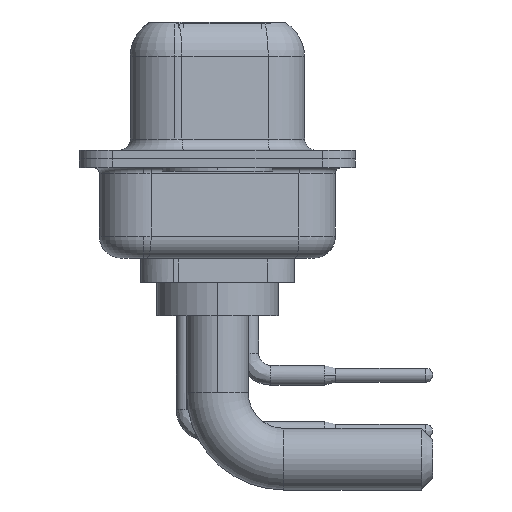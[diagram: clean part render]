
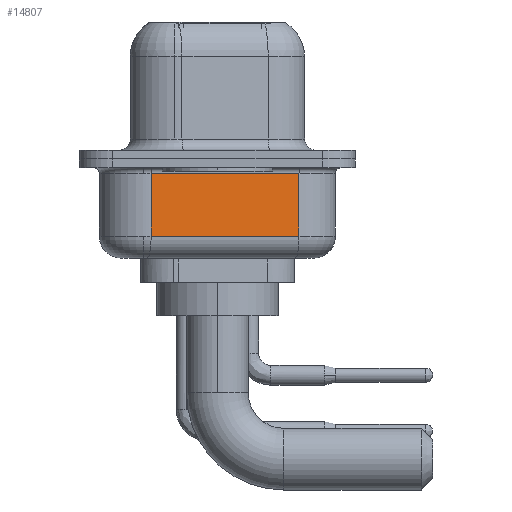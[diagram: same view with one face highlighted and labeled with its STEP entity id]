
A CAD part, left-side view. The second image highlights one B-rep face of the part: STEP entity #14807.
In plain terms, the highlighted planar face has unit normal (-0.985, -0.174, 0).
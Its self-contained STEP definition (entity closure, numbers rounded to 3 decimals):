
#488 = EDGE_CURVE ( 'NONE', #4602, #17712, #18403, .T. ) ;
#662 = LINE ( 'NONE', #10175, #16538 ) ;
#793 = AXIS2_PLACEMENT_3D ( 'NONE', #4955, #11199, #7824 ) ;
#2160 = CARTESIAN_POINT ( 'NONE',  ( 2.88, 3.003, -3.5 ) ) ;
#2682 = EDGE_CURVE ( 'NONE', #2698, #17712, #13853, .T. ) ;
#2698 = VERTEX_POINT ( 'NONE', #7511 ) ;
#3699 = LINE ( 'NONE', #5219, #5536 ) ;
#4392 = CARTESIAN_POINT ( 'NONE',  ( 2.88, 3.003, -4.5 ) ) ;
#4602 = VERTEX_POINT ( 'NONE', #2160 ) ;
#4955 = CARTESIAN_POINT ( 'NONE',  ( 2.88, 3.003, -4.5 ) ) ;
#4996 = CARTESIAN_POINT ( 'NONE',  ( 2.88, 3.003, -0.65 ) ) ;
#5219 = CARTESIAN_POINT ( 'NONE',  ( 2.88, 3.003, -3.5 ) ) ;
#5536 = VECTOR ( 'NONE', #17605, 1000. ) ;
#7511 = CARTESIAN_POINT ( 'NONE',  ( 4.062, -3.697, -0.65 ) ) ;
#7815 = EDGE_CURVE ( 'NONE', #4602, #18292, #3699, .T. ) ;
#7824 = DIRECTION ( 'NONE',  ( -0.174, 0.985, 0. ) ) ;
#8404 = ORIENTED_EDGE ( 'NONE', *, *, #7815, .T. ) ;
#9047 = DIRECTION ( 'NONE',  ( -0.174, 0.985, 0. ) ) ;
#10175 = CARTESIAN_POINT ( 'NONE',  ( 4.062, -3.697, -4.5 ) ) ;
#11102 = FACE_OUTER_BOUND ( 'NONE', #16351, .T. ) ;
#11199 = DIRECTION ( 'NONE',  ( 0.985, 0.174, 0. ) ) ;
#11299 = ORIENTED_EDGE ( 'NONE', *, *, #16924, .T. ) ;
#11946 = ORIENTED_EDGE ( 'NONE', *, *, #2682, .T. ) ;
#12136 = CARTESIAN_POINT ( 'NONE',  ( 2.88, 3.003, -0.65 ) ) ;
#13047 = DIRECTION ( 'NONE',  ( 0., 0., 1. ) ) ;
#13048 = CARTESIAN_POINT ( 'NONE',  ( 4.062, -3.697, -3.5 ) ) ;
#13853 = LINE ( 'NONE', #12136, #18129 ) ;
#14370 = PLANE ( 'NONE',  #793 ) ;
#14807 = ADVANCED_FACE ( 'NONE', ( #11102 ), #14370, .F. ) ;
#16351 = EDGE_LOOP ( 'NONE', ( #19496, #8404, #11299, #11946 ) ) ;
#16522 = VECTOR ( 'NONE', #16972, 1000. ) ;
#16538 = VECTOR ( 'NONE', #13047, 1000. ) ;
#16924 = EDGE_CURVE ( 'NONE', #18292, #2698, #662, .T. ) ;
#16972 = DIRECTION ( 'NONE',  ( 0., 0., 1. ) ) ;
#17605 = DIRECTION ( 'NONE',  ( 0.174, -0.985, 0. ) ) ;
#17712 = VERTEX_POINT ( 'NONE', #4996 ) ;
#18129 = VECTOR ( 'NONE', #9047, 1000. ) ;
#18292 = VERTEX_POINT ( 'NONE', #13048 ) ;
#18403 = LINE ( 'NONE', #4392, #16522 ) ;
#19496 = ORIENTED_EDGE ( 'NONE', *, *, #488, .F. ) ;
